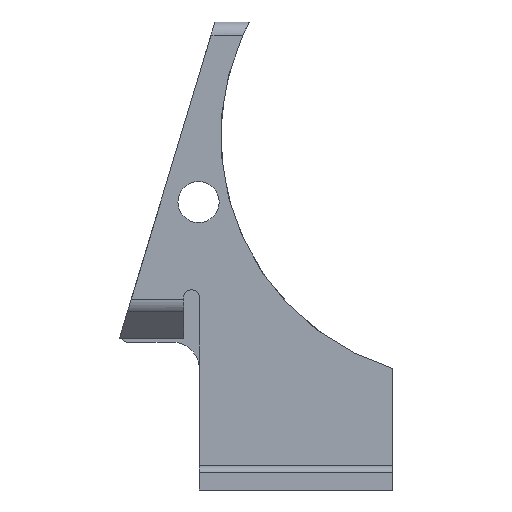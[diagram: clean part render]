
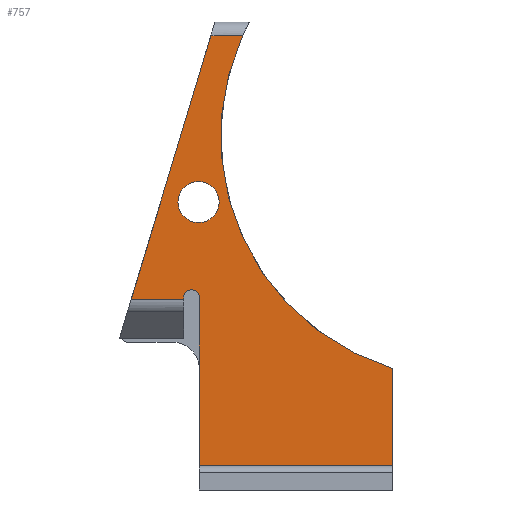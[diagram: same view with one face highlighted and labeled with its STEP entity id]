
A CAD part, left-side view. The second image highlights one B-rep face of the part: STEP entity #757.
In plain terms, the highlighted planar face has unit normal (-1, 0, 0).
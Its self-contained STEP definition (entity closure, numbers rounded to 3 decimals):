
#19=FACE_BOUND('',#91,.T.);
#25=PLANE('',#819);
#50=FACE_OUTER_BOUND('',#90,.T.);
#90=EDGE_LOOP('',(#536,#537,#538,#539,#540,#541,#542,#543,#544,#545,#546));
#91=EDGE_LOOP('',(#547));
#142=LINE('',#1127,#220);
#143=LINE('',#1130,#221);
#152=LINE('',#1155,#230);
#153=LINE('',#1159,#231);
#154=LINE('',#1163,#232);
#155=LINE('',#1165,#233);
#156=LINE('',#1167,#234);
#157=LINE('',#1170,#235);
#220=VECTOR('',#901,10.);
#221=VECTOR('',#904,10.);
#230=VECTOR('',#923,10.);
#231=VECTOR('',#926,10.);
#232=VECTOR('',#929,10.);
#233=VECTOR('',#930,10.);
#234=VECTOR('',#931,10.);
#235=VECTOR('',#934,10.);
#294=CIRCLE('',#820,0.5);
#295=CIRCLE('',#821,0.5);
#296=CIRCLE('',#822,17.951);
#297=CIRCLE('',#823,1.525);
#324=VERTEX_POINT('',#1120);
#327=VERTEX_POINT('',#1125);
#328=VERTEX_POINT('',#1129);
#339=VERTEX_POINT('',#1154);
#340=VERTEX_POINT('',#1156);
#341=VERTEX_POINT('',#1158);
#342=VERTEX_POINT('',#1160);
#343=VERTEX_POINT('',#1162);
#344=VERTEX_POINT('',#1164);
#345=VERTEX_POINT('',#1166);
#346=VERTEX_POINT('',#1168);
#347=VERTEX_POINT('',#1171);
#404=EDGE_CURVE('',#327,#324,#142,.T.);
#405=EDGE_CURVE('',#328,#324,#143,.T.);
#418=EDGE_CURVE('',#327,#339,#152,.T.);
#419=EDGE_CURVE('',#339,#340,#294,.T.);
#420=EDGE_CURVE('',#340,#341,#153,.T.);
#421=EDGE_CURVE('',#341,#342,#295,.T.);
#422=EDGE_CURVE('',#342,#343,#154,.T.);
#423=EDGE_CURVE('',#344,#343,#155,.T.);
#424=EDGE_CURVE('',#345,#344,#156,.T.);
#425=EDGE_CURVE('',#345,#346,#296,.T.);
#426=EDGE_CURVE('',#328,#346,#157,.T.);
#427=EDGE_CURVE('',#347,#347,#297,.T.);
#536=ORIENTED_EDGE('',*,*,#404,.F.);
#537=ORIENTED_EDGE('',*,*,#418,.T.);
#538=ORIENTED_EDGE('',*,*,#419,.T.);
#539=ORIENTED_EDGE('',*,*,#420,.T.);
#540=ORIENTED_EDGE('',*,*,#421,.T.);
#541=ORIENTED_EDGE('',*,*,#422,.T.);
#542=ORIENTED_EDGE('',*,*,#423,.F.);
#543=ORIENTED_EDGE('',*,*,#424,.F.);
#544=ORIENTED_EDGE('',*,*,#425,.T.);
#545=ORIENTED_EDGE('',*,*,#426,.F.);
#546=ORIENTED_EDGE('',*,*,#405,.T.);
#547=ORIENTED_EDGE('',*,*,#427,.T.);
#757=ADVANCED_FACE('',(#50,#19),#25,.T.);
#819=AXIS2_PLACEMENT_3D('',#1153,#921,#922);
#820=AXIS2_PLACEMENT_3D('',#1157,#924,#925);
#821=AXIS2_PLACEMENT_3D('',#1161,#927,#928);
#822=AXIS2_PLACEMENT_3D('',#1169,#932,#933);
#823=AXIS2_PLACEMENT_3D('',#1172,#935,#936);
#901=DIRECTION('',(0.,1.,0.));
#904=DIRECTION('',(0.,0.289,-0.957));
#921=DIRECTION('center_axis',(-1.,0.,0.));
#922=DIRECTION('ref_axis',(0.,0.,1.));
#923=DIRECTION('',(0.,0.,1.));
#924=DIRECTION('center_axis',(1.,0.,0.));
#925=DIRECTION('ref_axis',(0.,-1.,0.));
#926=DIRECTION('',(0.,-1.,0.));
#927=DIRECTION('center_axis',(1.,0.,0.));
#928=DIRECTION('ref_axis',(0.,-1.,0.));
#929=DIRECTION('',(0.,0.,-1.));
#930=DIRECTION('',(0.,1.,0.));
#931=DIRECTION('',(0.,0.,-1.));
#932=DIRECTION('center_axis',(1.,0.,0.));
#933=DIRECTION('ref_axis',(0.,-1.,0.));
#934=DIRECTION('',(0.,-1.,0.));
#935=DIRECTION('center_axis',(1.,0.,0.));
#936=DIRECTION('ref_axis',(0.,1.,0.));
#1120=CARTESIAN_POINT('',(-6.925,19.342,-19.231));
#1125=CARTESIAN_POINT('',(-6.925,15.45,-19.231));
#1127=CARTESIAN_POINT('',(-6.925,7.725,-19.231));
#1129=CARTESIAN_POINT('',(-6.925,13.442,0.3));
#1130=CARTESIAN_POINT('',(-6.925,17.207,-12.161));
#1153=CARTESIAN_POINT('Origin',(-6.925,0.,-32.05));
#1154=CARTESIAN_POINT('',(-6.925,15.45,-19.04));
#1155=CARTESIAN_POINT('',(-6.925,15.45,-25.795));
#1156=CARTESIAN_POINT('',(-6.925,14.95,-18.54));
#1157=CARTESIAN_POINT('Origin',(-6.925,14.95,-19.04));
#1158=CARTESIAN_POINT('',(-6.925,14.8,-18.54));
#1159=CARTESIAN_POINT('',(-6.925,7.475,-18.54));
#1160=CARTESIAN_POINT('',(-6.925,14.3,-19.04));
#1161=CARTESIAN_POINT('Origin',(-6.925,14.8,-19.04));
#1162=CARTESIAN_POINT('',(-6.925,14.3,-31.55));
#1163=CARTESIAN_POINT('',(-6.925,14.3,-27.225));
#1164=CARTESIAN_POINT('',(-6.925,0.,-31.55));
#1165=CARTESIAN_POINT('',(-6.925,0.,-31.55));
#1166=CARTESIAN_POINT('',(-6.925,0.,-24.35));
#1167=CARTESIAN_POINT('',(-6.925,0.,1.3));
#1168=CARTESIAN_POINT('',(-6.925,11.086,0.3));
#1169=CARTESIAN_POINT('Origin',(-6.925,-5.234,-7.178));
#1170=CARTESIAN_POINT('',(-6.925,0.,0.3));
#1171=CARTESIAN_POINT('',(-6.925,12.833,-12.038));
#1172=CARTESIAN_POINT('Origin',(-6.925,14.358,-12.038));
